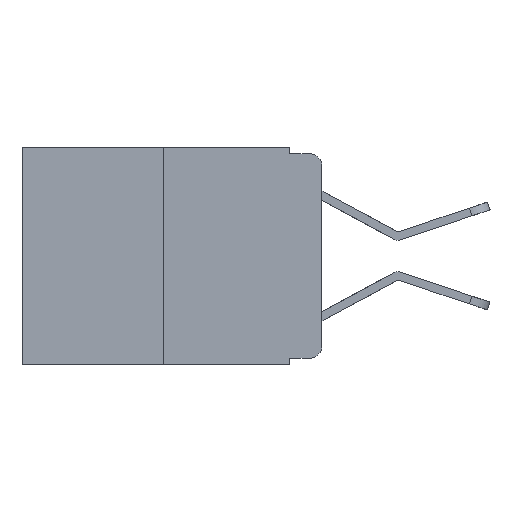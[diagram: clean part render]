
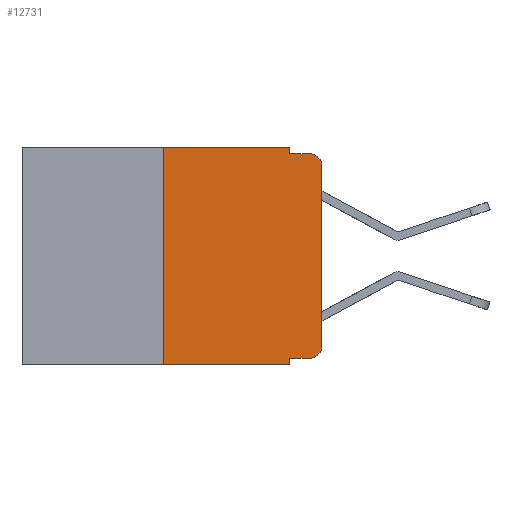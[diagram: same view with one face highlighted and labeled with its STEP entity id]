
A CAD part, left-side view. The second image highlights one B-rep face of the part: STEP entity #12731.
In plain terms, the highlighted planar face has unit normal (-1, 0, 0).
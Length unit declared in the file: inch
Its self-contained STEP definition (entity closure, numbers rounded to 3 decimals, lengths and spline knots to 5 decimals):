
#31 = VERTEX_POINT ( 'NONE', #8026 ) ;
#198 = ORIENTED_EDGE ( 'NONE', *, *, #2663, .F. ) ;
#273 = ORIENTED_EDGE ( 'NONE', *, *, #2111, .F. ) ;
#284 = ORIENTED_EDGE ( 'NONE', *, *, #4194, .T. ) ;
#301 = ORIENTED_EDGE ( 'NONE', *, *, #412, .F. ) ;
#412 = EDGE_CURVE ( 'NONE', #8843, #9154, #12763, .T. ) ;
#575 = ORIENTED_EDGE ( 'NONE', *, *, #4035, .T. ) ;
#806 = DIRECTION ( 'NONE',  ( 0., 0., 1. ) ) ;
#874 = ORIENTED_EDGE ( 'NONE', *, *, #1292, .F. ) ;
#884 = VERTEX_POINT ( 'NONE', #10691 ) ;
#1283 = ORIENTED_EDGE ( 'NONE', *, *, #12369, .F. ) ;
#1292 = EDGE_CURVE ( 'NONE', #6357, #31, #11720, .T. ) ;
#1728 = CARTESIAN_POINT ( 'NONE',  ( 0., 0.25, 0. ) ) ;
#1846 = EDGE_LOOP ( 'NONE', ( #2251, #7492, #198, #273, #1283, #874, #2429, #301, #284, #575 ) ) ;
#1886 = VERTEX_POINT ( 'NONE', #12225 ) ;
#1911 = EDGE_CURVE ( 'NONE', #6907, #884, #10117, .T. ) ;
#1952 = PLANE ( 'NONE',  #11726 ) ;
#2111 = EDGE_CURVE ( 'NONE', #5519, #1886, #3940, .T. ) ;
#2188 = LINE ( 'NONE', #3700, #4980 ) ;
#2251 = ORIENTED_EDGE ( 'NONE', *, *, #1911, .T. ) ;
#2429 = ORIENTED_EDGE ( 'NONE', *, *, #2777, .T. ) ;
#2584 = VERTEX_POINT ( 'NONE', #12940 ) ;
#2663 = EDGE_CURVE ( 'NONE', #1886, #9107, #7162, .T. ) ;
#2777 = EDGE_CURVE ( 'NONE', #6357, #9154, #9505, .T. ) ;
#3700 = CARTESIAN_POINT ( 'NONE',  ( 0., 0.473, 0. ) ) ;
#3862 = CARTESIAN_POINT ( 'NONE',  ( 0., 0., -0.313 ) ) ;
#3940 = LINE ( 'NONE', #9951, #5937 ) ;
#4035 = EDGE_CURVE ( 'NONE', #2584, #6907, #7634, .T. ) ;
#4076 = VECTOR ( 'NONE', #12535, 39.37008 ) ;
#4146 = CARTESIAN_POINT ( 'NONE',  ( 0., 0.473, 0. ) ) ;
#4194 = EDGE_CURVE ( 'NONE', #8843, #2584, #6603, .T. ) ;
#4212 = FACE_OUTER_BOUND ( 'NONE', #1846, .T. ) ;
#4456 = AXIS2_PLACEMENT_3D ( 'NONE', #10968, #5305, #11893 ) ;
#4470 = VECTOR ( 'NONE', #806, 39.37008 ) ;
#4743 = CARTESIAN_POINT ( 'NONE',  ( 0., 0.051, -0.333 ) ) ;
#4980 = VECTOR ( 'NONE', #9501, 39.37008 ) ;
#5137 = DIRECTION ( 'NONE',  ( 0., 0., -1. ) ) ;
#5297 = CARTESIAN_POINT ( 'NONE',  ( 0., 0.02, -0.03 ) ) ;
#5305 = DIRECTION ( 'NONE',  ( -1., 0., 0. ) ) ;
#5519 = VERTEX_POINT ( 'NONE', #7545 ) ;
#5937 = VECTOR ( 'NONE', #10469, 39.37008 ) ;
#5971 = VECTOR ( 'NONE', #12265, 39.37008 ) ;
#5982 = CARTESIAN_POINT ( 'NONE',  ( 0., 0.25, -0.343 ) ) ;
#6270 = DIRECTION ( 'NONE',  ( 0., 0., -1. ) ) ;
#6357 = VERTEX_POINT ( 'NONE', #5982 ) ;
#6603 = LINE ( 'NONE', #4743, #5971 ) ;
#6907 = VERTEX_POINT ( 'NONE', #3862 ) ;
#7162 = LINE ( 'NONE', #11890, #11812 ) ;
#7270 = EDGE_CURVE ( 'NONE', #884, #9107, #11645, .T. ) ;
#7492 = ORIENTED_EDGE ( 'NONE', *, *, #7270, .T. ) ;
#7545 = CARTESIAN_POINT ( 'NONE',  ( 0., 0.051, 0. ) ) ;
#7634 = CIRCLE ( 'NONE', #4456, 0.02 ) ;
#8026 = CARTESIAN_POINT ( 'NONE',  ( 0., 0.25, 0. ) ) ;
#8843 = VERTEX_POINT ( 'NONE', #12196 ) ;
#9107 = VERTEX_POINT ( 'NONE', #12429 ) ;
#9154 = VERTEX_POINT ( 'NONE', #12470 ) ;
#9501 = DIRECTION ( 'NONE',  ( 0., -1., 0. ) ) ;
#9505 = LINE ( 'NONE', #12406, #4076 ) ;
#9521 = CARTESIAN_POINT ( 'NONE',  ( 0., 0.051, 0. ) ) ;
#9951 = CARTESIAN_POINT ( 'NONE',  ( 0., 0.051, 0. ) ) ;
#10117 = LINE ( 'NONE', #10933, #12845 ) ;
#10469 = DIRECTION ( 'NONE',  ( 0., 0., -1. ) ) ;
#10691 = CARTESIAN_POINT ( 'NONE',  ( 0., 0., -0.03 ) ) ;
#10824 = DIRECTION ( 'NONE',  ( 1., 0., 0. ) ) ;
#10933 = CARTESIAN_POINT ( 'NONE',  ( 0., 0., 0. ) ) ;
#10968 = CARTESIAN_POINT ( 'NONE',  ( 0., 0.02, -0.313 ) ) ;
#11553 = AXIS2_PLACEMENT_3D ( 'NONE', #5297, #11885, #6270 ) ;
#11645 = CIRCLE ( 'NONE', #11553, 0.02 ) ;
#11720 = LINE ( 'NONE', #1728, #4470 ) ;
#11726 = AXIS2_PLACEMENT_3D ( 'NONE', #4146, #10824, #5137 ) ;
#11812 = VECTOR ( 'NONE', #12034, 39.37008 ) ;
#11885 = DIRECTION ( 'NONE',  ( -1., 0., 0. ) ) ;
#11890 = CARTESIAN_POINT ( 'NONE',  ( 0., 0.051, -0.01 ) ) ;
#11893 = DIRECTION ( 'NONE',  ( 0., 0., -1. ) ) ;
#12034 = DIRECTION ( 'NONE',  ( 0., -1., 0. ) ) ;
#12196 = CARTESIAN_POINT ( 'NONE',  ( 0., 0.051, -0.333 ) ) ;
#12225 = CARTESIAN_POINT ( 'NONE',  ( 0., 0.051, -0.01 ) ) ;
#12265 = DIRECTION ( 'NONE',  ( 0., -1., 0. ) ) ;
#12266 = DIRECTION ( 'NONE',  ( 0., 0., 1. ) ) ;
#12369 = EDGE_CURVE ( 'NONE', #31, #5519, #2188, .T. ) ;
#12406 = CARTESIAN_POINT ( 'NONE',  ( 0., 0.473, -0.343 ) ) ;
#12429 = CARTESIAN_POINT ( 'NONE',  ( 0., 0.02, -0.01 ) ) ;
#12470 = CARTESIAN_POINT ( 'NONE',  ( 0., 0.051, -0.343 ) ) ;
#12480 = VECTOR ( 'NONE', #12553, 39.37008 ) ;
#12535 = DIRECTION ( 'NONE',  ( 0., -1., 0. ) ) ;
#12553 = DIRECTION ( 'NONE',  ( 0., 0., -1. ) ) ;
#12731 = ADVANCED_FACE ( 'NONE', ( #4212 ), #1952, .F. ) ;
#12763 = LINE ( 'NONE', #9521, #12480 ) ;
#12845 = VECTOR ( 'NONE', #12266, 39.37008 ) ;
#12940 = CARTESIAN_POINT ( 'NONE',  ( 0., 0.02, -0.333 ) ) ;
